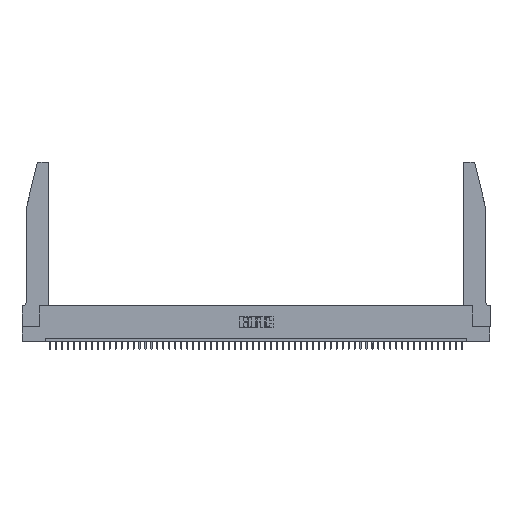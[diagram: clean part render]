
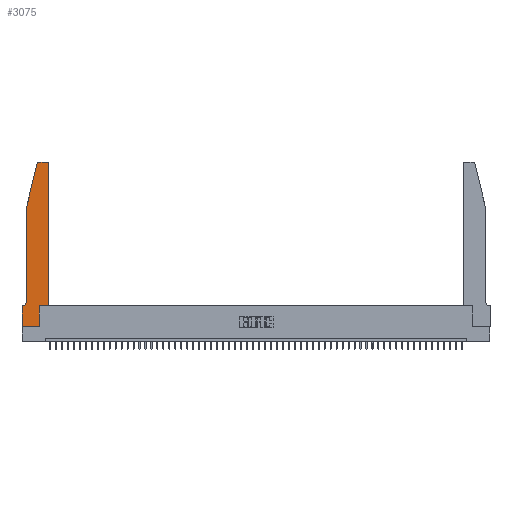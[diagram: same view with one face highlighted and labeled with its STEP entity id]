
A CAD part, top view. The second image highlights one B-rep face of the part: STEP entity #3075.
In plain terms, the highlighted planar face has unit normal (0, 0, 1).
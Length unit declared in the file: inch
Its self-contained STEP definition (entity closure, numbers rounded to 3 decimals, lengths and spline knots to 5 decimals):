
#274 = CARTESIAN_POINT ( 'NONE',  ( 0., 0.35, 0.37 ) ) ;
#1073 = EDGE_CURVE ( 'NONE', #30544, #21436, #31321, .T. ) ;
#1819 = AXIS2_PLACEMENT_3D ( 'NONE', #14908, #19265, #48093 ) ;
#1833 = CARTESIAN_POINT ( 'NONE',  ( 0.25487, 2.72718, 0.37 ) ) ;
#1856 = FACE_OUTER_BOUND ( 'NONE', #41582, .T. ) ;
#3075 = ADVANCED_FACE ( 'NONE', ( #1856 ), #27688, .T. ) ;
#3723 = CARTESIAN_POINT ( 'NONE',  ( 0.284, 2.72, 0.37 ) ) ;
#4191 = CARTESIAN_POINT ( 'NONE',  ( 0.0755, 0.35, 0.37 ) ) ;
#4324 = AXIS2_PLACEMENT_3D ( 'NONE', #9484, #50828, #17930 ) ;
#5019 = VERTEX_POINT ( 'NONE', #18862 ) ;
#5263 = VERTEX_POINT ( 'NONE', #33759 ) ;
#5870 = EDGE_CURVE ( 'NONE', #29860, #5019, #14062, .T. ) ;
#6024 = EDGE_CURVE ( 'NONE', #45079, #30544, #20006, .T. ) ;
#6349 = CARTESIAN_POINT ( 'NONE',  ( 0.2605, 2.75, 0.37 ) ) ;
#6637 = VERTEX_POINT ( 'NONE', #31023 ) ;
#7422 = AXIS2_PLACEMENT_3D ( 'NONE', #45343, #40702, #12145 ) ;
#8235 = VERTEX_POINT ( 'NONE', #14369 ) ;
#8464 = EDGE_CURVE ( 'NONE', #6637, #5263, #52205, .T. ) ;
#8843 = ORIENTED_EDGE ( 'NONE', *, *, #8464, .T. ) ;
#8948 = EDGE_CURVE ( 'NONE', #21436, #6637, #45548, .T. ) ;
#9484 = CARTESIAN_POINT ( 'NONE',  ( 0.0055, 0.42, 0.37 ) ) ;
#9823 = EDGE_CURVE ( 'NONE', #42692, #11919, #30570, .T. ) ;
#10374 = ORIENTED_EDGE ( 'NONE', *, *, #24179, .T. ) ;
#10654 = DIRECTION ( 'NONE',  ( 1., 0., 0. ) ) ;
#11817 = CARTESIAN_POINT ( 'NONE',  ( 0.4505, 0.35, 0.37 ) ) ;
#11919 = VERTEX_POINT ( 'NONE', #1833 ) ;
#12145 = DIRECTION ( 'NONE',  ( 1., 0., 0. ) ) ;
#13301 = ORIENTED_EDGE ( 'NONE', *, *, #18457, .T. ) ;
#13681 = VECTOR ( 'NONE', #52891, 39.37008 ) ;
#14001 = CARTESIAN_POINT ( 'NONE',  ( 0., 0., 0.37 ) ) ;
#14062 = LINE ( 'NONE', #35813, #19734 ) ;
#14369 = CARTESIAN_POINT ( 'NONE',  ( 0.0055, 0.35, 0.37 ) ) ;
#14796 = DIRECTION ( 'NONE',  ( -0.239, -0.971, 0. ) ) ;
#14800 = DIRECTION ( 'NONE',  ( 0., -1., 0. ) ) ;
#14908 = CARTESIAN_POINT ( 'NONE',  ( 0.4205, 2.72, 0.37 ) ) ;
#15377 = CARTESIAN_POINT ( 'NONE',  ( 0.2865, 0.35, 0.37 ) ) ;
#15419 = CARTESIAN_POINT ( 'NONE',  ( 0.2865, 0., 0.37 ) ) ;
#16715 = DIRECTION ( 'NONE',  ( 0., 1., 0. ) ) ;
#16803 = EDGE_CURVE ( 'NONE', #5019, #8235, #32975, .T. ) ;
#17810 = LINE ( 'NONE', #14001, #39499 ) ;
#17930 = DIRECTION ( 'NONE',  ( -1., 0., 0. ) ) ;
#18370 = ORIENTED_EDGE ( 'NONE', *, *, #6024, .T. ) ;
#18416 = AXIS2_PLACEMENT_3D ( 'NONE', #3723, #41251, #45076 ) ;
#18457 = EDGE_CURVE ( 'NONE', #11919, #29860, #52561, .T. ) ;
#18631 = ORIENTED_EDGE ( 'NONE', *, *, #16803, .T. ) ;
#18862 = CARTESIAN_POINT ( 'NONE',  ( 0.0755, 0.42, 0.37 ) ) ;
#19265 = DIRECTION ( 'NONE',  ( 0., 0., 1. ) ) ;
#19734 = VECTOR ( 'NONE', #47774, 39.37008 ) ;
#20006 = LINE ( 'NONE', #15377, #13681 ) ;
#20540 = DIRECTION ( 'NONE',  ( -1., 0., 0. ) ) ;
#21436 = VERTEX_POINT ( 'NONE', #42579 ) ;
#21700 = VECTOR ( 'NONE', #14796, 39.37008 ) ;
#22949 = DIRECTION ( 'NONE',  ( -1., 0., 0. ) ) ;
#23375 = CARTESIAN_POINT ( 'NONE',  ( 0.2865, 0.35, 0.37 ) ) ;
#24179 = EDGE_CURVE ( 'NONE', #8235, #52305, #25701, .T. ) ;
#24350 = EDGE_CURVE ( 'NONE', #52305, #26095, #17810, .T. ) ;
#25701 = LINE ( 'NONE', #4191, #47428 ) ;
#26095 = VERTEX_POINT ( 'NONE', #37012 ) ;
#27688 = PLANE ( 'NONE',  #7422 ) ;
#27742 = ORIENTED_EDGE ( 'NONE', *, *, #24350, .T. ) ;
#27870 = CARTESIAN_POINT ( 'NONE',  ( 0.0755, 2., 0.37 ) ) ;
#29200 = LINE ( 'NONE', #53651, #40025 ) ;
#29385 = ORIENTED_EDGE ( 'NONE', *, *, #39863, .T. ) ;
#29860 = VERTEX_POINT ( 'NONE', #27870 ) ;
#30527 = VECTOR ( 'NONE', #16715, 39.37008 ) ;
#30544 = VERTEX_POINT ( 'NONE', #23375 ) ;
#30570 = CIRCLE ( 'NONE', #18416, 0.03 ) ;
#31023 = CARTESIAN_POINT ( 'NONE',  ( 0.4505, 2.72, 0.37 ) ) ;
#31321 = LINE ( 'NONE', #47913, #53334 ) ;
#32823 = EDGE_CURVE ( 'NONE', #26095, #45079, #29200, .T. ) ;
#32975 = CIRCLE ( 'NONE', #4324, 0.07 ) ;
#33759 = CARTESIAN_POINT ( 'NONE',  ( 0.4205, 2.75, 0.37 ) ) ;
#35703 = CARTESIAN_POINT ( 'NONE',  ( 0.284, 2.75, 0.37 ) ) ;
#35813 = CARTESIAN_POINT ( 'NONE',  ( 0.0755, 2., 0.37 ) ) ;
#37012 = CARTESIAN_POINT ( 'NONE',  ( 0., 0., 0.37 ) ) ;
#39499 = VECTOR ( 'NONE', #14800, 39.37008 ) ;
#39863 = EDGE_CURVE ( 'NONE', #5263, #42692, #47677, .T. ) ;
#40025 = VECTOR ( 'NONE', #50395, 39.37008 ) ;
#40702 = DIRECTION ( 'NONE',  ( 0., 0., 1. ) ) ;
#41251 = DIRECTION ( 'NONE',  ( 0., 0., 1. ) ) ;
#41582 = EDGE_LOOP ( 'NONE', ( #29385, #44060, #13301, #53728, #18631, #10374, #27742, #44767, #18370, #41752, #44886, #8843 ) ) ;
#41752 = ORIENTED_EDGE ( 'NONE', *, *, #1073, .T. ) ;
#42579 = CARTESIAN_POINT ( 'NONE',  ( 0.4505, 0.35, 0.37 ) ) ;
#42692 = VERTEX_POINT ( 'NONE', #35703 ) ;
#44060 = ORIENTED_EDGE ( 'NONE', *, *, #9823, .T. ) ;
#44439 = CARTESIAN_POINT ( 'NONE',  ( 0.0755, 2., 0.37 ) ) ;
#44767 = ORIENTED_EDGE ( 'NONE', *, *, #32823, .T. ) ;
#44886 = ORIENTED_EDGE ( 'NONE', *, *, #8948, .T. ) ;
#45076 = DIRECTION ( 'NONE',  ( 1., 0., 0. ) ) ;
#45079 = VERTEX_POINT ( 'NONE', #15419 ) ;
#45343 = CARTESIAN_POINT ( 'NONE',  ( 0., 0.35, 0.37 ) ) ;
#45548 = LINE ( 'NONE', #11817, #30527 ) ;
#47428 = VECTOR ( 'NONE', #20540, 39.37008 ) ;
#47677 = LINE ( 'NONE', #6349, #52813 ) ;
#47774 = DIRECTION ( 'NONE',  ( 0., -1., 0. ) ) ;
#47913 = CARTESIAN_POINT ( 'NONE',  ( 0.4505, 0.35, 0.37 ) ) ;
#48093 = DIRECTION ( 'NONE',  ( 1., 0., 0. ) ) ;
#50395 = DIRECTION ( 'NONE',  ( 1., 0., 0. ) ) ;
#50828 = DIRECTION ( 'NONE',  ( 0., 0., -1. ) ) ;
#52205 = CIRCLE ( 'NONE', #1819, 0.03 ) ;
#52305 = VERTEX_POINT ( 'NONE', #274 ) ;
#52561 = LINE ( 'NONE', #44439, #21700 ) ;
#52813 = VECTOR ( 'NONE', #22949, 39.37008 ) ;
#52891 = DIRECTION ( 'NONE',  ( 0., 1., 0. ) ) ;
#53334 = VECTOR ( 'NONE', #10654, 39.37008 ) ;
#53651 = CARTESIAN_POINT ( 'NONE',  ( 0., 0., 0.37 ) ) ;
#53728 = ORIENTED_EDGE ( 'NONE', *, *, #5870, .T. ) ;
